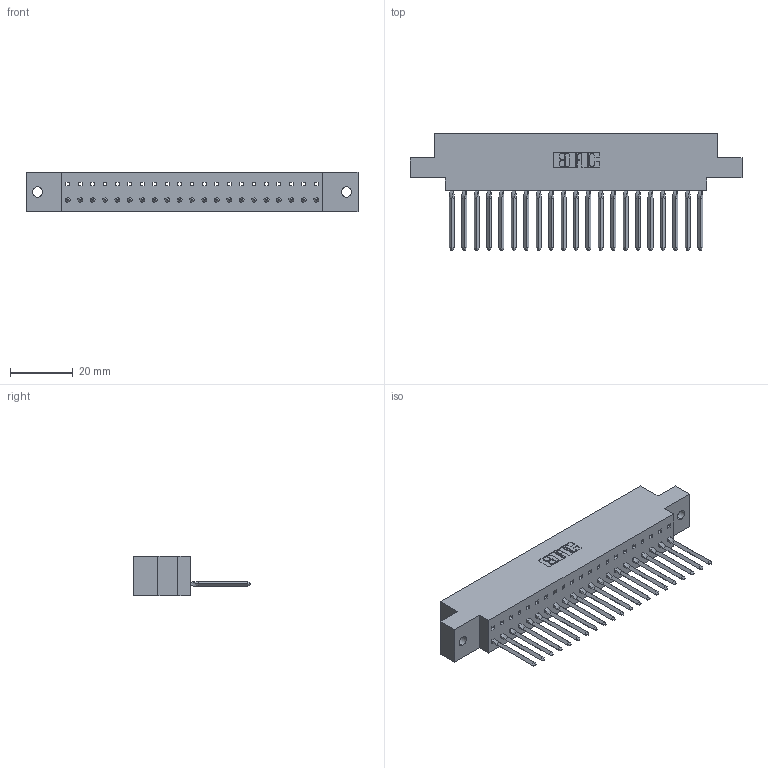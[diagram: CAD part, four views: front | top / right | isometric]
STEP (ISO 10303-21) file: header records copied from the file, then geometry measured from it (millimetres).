
FILE_DESCRIPTION (( 'STEP AP203' ), '1' );
FILE_NAME ('317-021-542-602.STEP', '2020-02-27T16:57:10', ( '' ), ( '' ), 'SwSTEP 2.0', 'SolidWorks 2016', '' );
FILE_SCHEMA (( 'CONFIG_CONTROL_DESIGN' ));
Length unit declared in the file: inch
Products named in the file (3): 317-021-542-602; 317 Part_.144 Dia; 317-290-003_542
Assembly tree (22 placements, depth 2):
  317-021-542-602
    317 Part_.144 Dia
    317-290-003_542  x21
Bounding box: 105.92 x 37.34 x 12.7 mm (x, y, z)
Volume: 15766.4 mm3; surface area: 18491.9 mm2
Topology: 22 solids, 22 shells, 1677 faces, 4832 edges, 3122 vertices
Faces by surface type: plane 1402, cylinder 191, bspline 84
Entity records: 31633 total; most frequent: CARTESIAN_POINT 5860, ORIENTED_EDGE 5544, DIRECTION 4658, EDGE_CURVE 2772, VECTOR 2602, LINE 2602, VERTEX_POINT 1842, AXIS2_PLACEMENT_3D 1028
